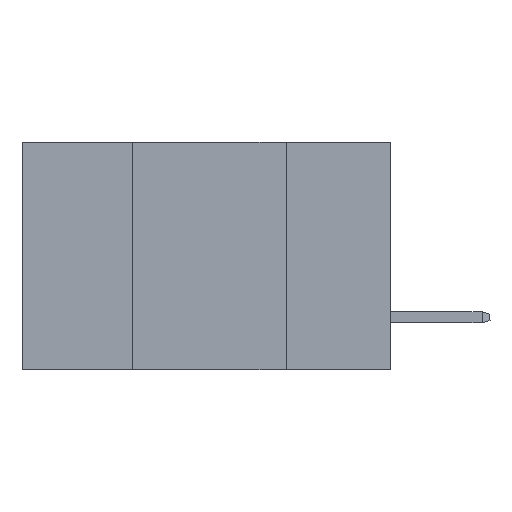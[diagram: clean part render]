
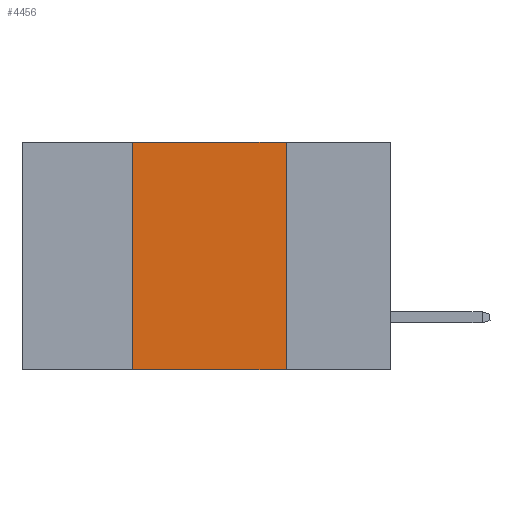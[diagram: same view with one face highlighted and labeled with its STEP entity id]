
A CAD part, left-side view. The second image highlights one B-rep face of the part: STEP entity #4456.
In plain terms, the highlighted planar face has unit normal (-1, 0, 0).
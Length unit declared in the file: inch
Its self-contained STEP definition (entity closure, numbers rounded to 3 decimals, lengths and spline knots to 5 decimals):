
#149 = VERTEX_POINT ( 'NONE', #6888 ) ;
#259 = CARTESIAN_POINT ( 'NONE',  ( 0., 0.17, -0.37 ) ) ;
#380 = ORIENTED_EDGE ( 'NONE', *, *, #4648, .F. ) ;
#574 = CARTESIAN_POINT ( 'NONE',  ( 0., 0.17, 0. ) ) ;
#738 = VECTOR ( 'NONE', #6710, 39.37008 ) ;
#1000 = VECTOR ( 'NONE', #4454, 39.37008 ) ;
#2066 = VECTOR ( 'NONE', #9025, 39.37008 ) ;
#2655 = DIRECTION ( 'NONE',  ( 0., 0., -1. ) ) ;
#2697 = ORIENTED_EDGE ( 'NONE', *, *, #6451, .F. ) ;
#2797 = DIRECTION ( 'NONE',  ( 1., 0., 0. ) ) ;
#2852 = DIRECTION ( 'NONE',  ( 0., 0., -1. ) ) ;
#2873 = PLANE ( 'NONE',  #7363 ) ;
#3161 = ORIENTED_EDGE ( 'NONE', *, *, #7770, .T. ) ;
#3347 = EDGE_CURVE ( 'NONE', #7887, #149, #8732, .T. ) ;
#3433 = FACE_OUTER_BOUND ( 'NONE', #10009, .T. ) ;
#3752 = CARTESIAN_POINT ( 'NONE',  ( 0., 0.6, 0. ) ) ;
#3873 = ORIENTED_EDGE ( 'NONE', *, *, #3347, .F. ) ;
#3959 = VERTEX_POINT ( 'NONE', #259 ) ;
#4349 = CARTESIAN_POINT ( 'NONE',  ( 0., 0.17, 0. ) ) ;
#4422 = CARTESIAN_POINT ( 'NONE',  ( 0., 0.6, 0. ) ) ;
#4453 = CARTESIAN_POINT ( 'NONE',  ( 0., 0.42, 0. ) ) ;
#4454 = DIRECTION ( 'NONE',  ( 0., -1., 0. ) ) ;
#4456 = ADVANCED_FACE ( 'NONE', ( #3433 ), #2873, .F. ) ;
#4648 = EDGE_CURVE ( 'NONE', #7650, #3959, #4962, .T. ) ;
#4962 = LINE ( 'NONE', #4349, #6819 ) ;
#6409 = LINE ( 'NONE', #8137, #2066 ) ;
#6451 = EDGE_CURVE ( 'NONE', #149, #7650, #7474, .T. ) ;
#6710 = DIRECTION ( 'NONE',  ( 0., 0., 1. ) ) ;
#6819 = VECTOR ( 'NONE', #2655, 39.37008 ) ;
#6888 = CARTESIAN_POINT ( 'NONE',  ( 0., 0.42, 0. ) ) ;
#7363 = AXIS2_PLACEMENT_3D ( 'NONE', #3752, #2797, #2852 ) ;
#7474 = LINE ( 'NONE', #4422, #1000 ) ;
#7650 = VERTEX_POINT ( 'NONE', #574 ) ;
#7770 = EDGE_CURVE ( 'NONE', #7887, #3959, #6409, .T. ) ;
#7887 = VERTEX_POINT ( 'NONE', #10007 ) ;
#8137 = CARTESIAN_POINT ( 'NONE',  ( 0., 0.6, -0.37 ) ) ;
#8732 = LINE ( 'NONE', #4453, #738 ) ;
#9025 = DIRECTION ( 'NONE',  ( 0., -1., 0. ) ) ;
#10007 = CARTESIAN_POINT ( 'NONE',  ( 0., 0.42, -0.37 ) ) ;
#10009 = EDGE_LOOP ( 'NONE', ( #380, #2697, #3873, #3161 ) ) ;
